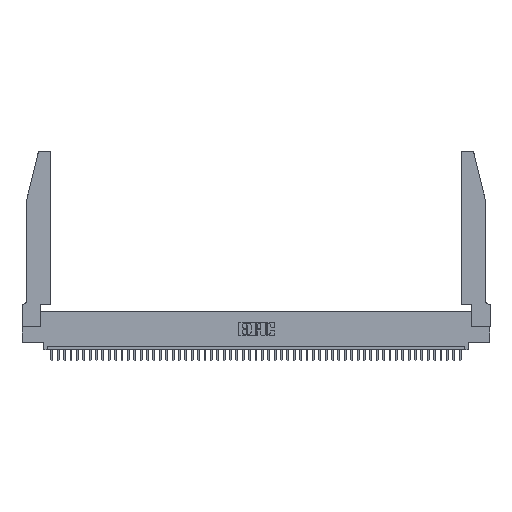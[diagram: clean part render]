
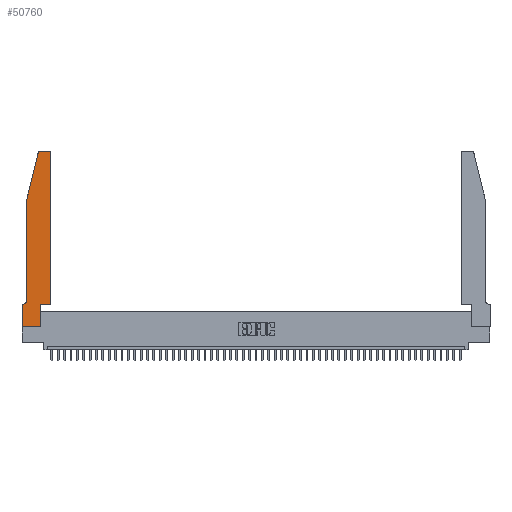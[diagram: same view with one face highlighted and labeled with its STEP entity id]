
A CAD part, top view. The second image highlights one B-rep face of the part: STEP entity #50760.
In plain terms, the highlighted planar face has unit normal (0, 0, 1).
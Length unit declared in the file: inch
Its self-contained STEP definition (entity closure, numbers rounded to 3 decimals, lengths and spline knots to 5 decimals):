
#1362 = CARTESIAN_POINT ( 'NONE',  ( 0.2605, 2.75, 0.37 ) ) ;
#1444 = AXIS2_PLACEMENT_3D ( 'NONE', #28934, #48845, #25145 ) ;
#1711 = CARTESIAN_POINT ( 'NONE',  ( 0.0055, 0.35, 0.37 ) ) ;
#2375 = VECTOR ( 'NONE', #44565, 39.37008 ) ;
#2603 = VERTEX_POINT ( 'NONE', #12487 ) ;
#3079 = VERTEX_POINT ( 'NONE', #20171 ) ;
#3161 = ORIENTED_EDGE ( 'NONE', *, *, #40107, .T. ) ;
#3470 = VECTOR ( 'NONE', #37490, 39.37008 ) ;
#3906 = VERTEX_POINT ( 'NONE', #20942 ) ;
#4210 = CARTESIAN_POINT ( 'NONE',  ( 0.25487, 2.72718, 0.37 ) ) ;
#4212 = ORIENTED_EDGE ( 'NONE', *, *, #50804, .T. ) ;
#4453 = ORIENTED_EDGE ( 'NONE', *, *, #38743, .T. ) ;
#4832 = DIRECTION ( 'NONE',  ( -0.239, -0.971, 0. ) ) ;
#5018 = CARTESIAN_POINT ( 'NONE',  ( 0.0755, 0.35, 0.37 ) ) ;
#5999 = LINE ( 'NONE', #22729, #45299 ) ;
#7219 = DIRECTION ( 'NONE',  ( 1., 0., 0. ) ) ;
#7527 = CARTESIAN_POINT ( 'NONE',  ( 0.2865, 0.35, 0.37 ) ) ;
#7775 = LINE ( 'NONE', #41407, #3470 ) ;
#7816 = VERTEX_POINT ( 'NONE', #7527 ) ;
#8596 = EDGE_CURVE ( 'NONE', #30933, #3079, #15545, .T. ) ;
#8912 = ORIENTED_EDGE ( 'NONE', *, *, #29137, .T. ) ;
#9221 = VERTEX_POINT ( 'NONE', #22425 ) ;
#9633 = CARTESIAN_POINT ( 'NONE',  ( 0.284, 2.72, 0.37 ) ) ;
#12421 = ORIENTED_EDGE ( 'NONE', *, *, #32654, .T. ) ;
#12487 = CARTESIAN_POINT ( 'NONE',  ( 0.2865, 0., 0.37 ) ) ;
#13029 = CARTESIAN_POINT ( 'NONE',  ( 0.4205, 2.72, 0.37 ) ) ;
#13188 = DIRECTION ( 'NONE',  ( 0., 0., 1. ) ) ;
#13356 = DIRECTION ( 'NONE',  ( 1., 0., 0. ) ) ;
#13885 = DIRECTION ( 'NONE',  ( 0., 0., 1. ) ) ;
#14765 = CARTESIAN_POINT ( 'NONE',  ( 0., 0.35, 0.37 ) ) ;
#14926 = EDGE_CURVE ( 'NONE', #9221, #30933, #44892, .T. ) ;
#15184 = DIRECTION ( 'NONE',  ( 0., -1., 0. ) ) ;
#15196 = VECTOR ( 'NONE', #15184, 39.37008 ) ;
#15411 = AXIS2_PLACEMENT_3D ( 'NONE', #9633, #13885, #41027 ) ;
#15545 = LINE ( 'NONE', #28526, #48084 ) ;
#15895 = VECTOR ( 'NONE', #19348, 39.37008 ) ;
#16087 = VERTEX_POINT ( 'NONE', #37648 ) ;
#16365 = DIRECTION ( 'NONE',  ( -1., 0., 0. ) ) ;
#16500 = LINE ( 'NONE', #1362, #29383 ) ;
#17758 = FACE_OUTER_BOUND ( 'NONE', #36509, .T. ) ;
#18768 = VERTEX_POINT ( 'NONE', #48513 ) ;
#18988 = DIRECTION ( 'NONE',  ( 0., 1., 0. ) ) ;
#19348 = DIRECTION ( 'NONE',  ( 1., 0., 0. ) ) ;
#19803 = ORIENTED_EDGE ( 'NONE', *, *, #22388, .T. ) ;
#20152 = VERTEX_POINT ( 'NONE', #38486 ) ;
#20171 = CARTESIAN_POINT ( 'NONE',  ( 0.0755, 2., 0.37 ) ) ;
#20942 = CARTESIAN_POINT ( 'NONE',  ( 0., 0.35, 0.37 ) ) ;
#21685 = LINE ( 'NONE', #42361, #37066 ) ;
#22388 = EDGE_CURVE ( 'NONE', #34232, #47552, #23246, .T. ) ;
#22425 = CARTESIAN_POINT ( 'NONE',  ( 0.284, 2.75, 0.37 ) ) ;
#22729 = CARTESIAN_POINT ( 'NONE',  ( 0.0755, 2., 0.37 ) ) ;
#23246 = LINE ( 'NONE', #36686, #2375 ) ;
#23311 = DIRECTION ( 'NONE',  ( 0., 0., 1. ) ) ;
#23414 = CARTESIAN_POINT ( 'NONE',  ( 0.4505, 2.72, 0.37 ) ) ;
#25145 = DIRECTION ( 'NONE',  ( -1., 0., 0. ) ) ;
#26842 = CARTESIAN_POINT ( 'NONE',  ( 0., 0., 0.37 ) ) ;
#27106 = PLANE ( 'NONE',  #31131 ) ;
#28047 = EDGE_CURVE ( 'NONE', #18768, #9221, #16500, .T. ) ;
#28526 = CARTESIAN_POINT ( 'NONE',  ( 0.0755, 2., 0.37 ) ) ;
#28934 = CARTESIAN_POINT ( 'NONE',  ( 0.0055, 0.42, 0.37 ) ) ;
#29137 = EDGE_CURVE ( 'NONE', #3906, #16087, #29869, .T. ) ;
#29383 = VECTOR ( 'NONE', #44754, 39.37008 ) ;
#29869 = LINE ( 'NONE', #26842, #15196 ) ;
#30098 = ORIENTED_EDGE ( 'NONE', *, *, #8596, .T. ) ;
#30838 = ORIENTED_EDGE ( 'NONE', *, *, #46877, .T. ) ;
#30933 = VERTEX_POINT ( 'NONE', #4210 ) ;
#31131 = AXIS2_PLACEMENT_3D ( 'NONE', #14765, #23311, #7219 ) ;
#31739 = CIRCLE ( 'NONE', #44949, 0.03 ) ;
#31907 = LINE ( 'NONE', #5018, #42383 ) ;
#32654 = EDGE_CURVE ( 'NONE', #47552, #18768, #31739, .T. ) ;
#34232 = VERTEX_POINT ( 'NONE', #38812 ) ;
#34559 = DIRECTION ( 'NONE',  ( 0., -1., 0. ) ) ;
#35914 = ORIENTED_EDGE ( 'NONE', *, *, #28047, .T. ) ;
#36509 = EDGE_LOOP ( 'NONE', ( #35914, #39412, #30098, #30838, #3161, #4453, #8912, #43967, #37861, #4212, #19803, #12421 ) ) ;
#36686 = CARTESIAN_POINT ( 'NONE',  ( 0.4505, 0.35, 0.37 ) ) ;
#37066 = VECTOR ( 'NONE', #18988, 39.37008 ) ;
#37326 = EDGE_CURVE ( 'NONE', #2603, #7816, #21685, .T. ) ;
#37490 = DIRECTION ( 'NONE',  ( 1., 0., 0. ) ) ;
#37648 = CARTESIAN_POINT ( 'NONE',  ( 0., 0., 0.37 ) ) ;
#37861 = ORIENTED_EDGE ( 'NONE', *, *, #37326, .T. ) ;
#38486 = CARTESIAN_POINT ( 'NONE',  ( 0.0755, 0.42, 0.37 ) ) ;
#38743 = EDGE_CURVE ( 'NONE', #48579, #3906, #31907, .T. ) ;
#38812 = CARTESIAN_POINT ( 'NONE',  ( 0.4505, 0.35, 0.37 ) ) ;
#38981 = CARTESIAN_POINT ( 'NONE',  ( 0.4505, 0.35, 0.37 ) ) ;
#39412 = ORIENTED_EDGE ( 'NONE', *, *, #14926, .T. ) ;
#40107 = EDGE_CURVE ( 'NONE', #20152, #48579, #45900, .T. ) ;
#40837 = EDGE_CURVE ( 'NONE', #16087, #2603, #7775, .T. ) ;
#41027 = DIRECTION ( 'NONE',  ( 1., 0., 0. ) ) ;
#41407 = CARTESIAN_POINT ( 'NONE',  ( 0., 0., 0.37 ) ) ;
#42361 = CARTESIAN_POINT ( 'NONE',  ( 0.2865, 0.35, 0.37 ) ) ;
#42383 = VECTOR ( 'NONE', #16365, 39.37008 ) ;
#43967 = ORIENTED_EDGE ( 'NONE', *, *, #40837, .T. ) ;
#44565 = DIRECTION ( 'NONE',  ( 0., 1., 0. ) ) ;
#44754 = DIRECTION ( 'NONE',  ( -1., 0., 0. ) ) ;
#44892 = CIRCLE ( 'NONE', #15411, 0.03 ) ;
#44949 = AXIS2_PLACEMENT_3D ( 'NONE', #13029, #13188, #13356 ) ;
#45299 = VECTOR ( 'NONE', #34559, 39.37008 ) ;
#45900 = CIRCLE ( 'NONE', #1444, 0.07 ) ;
#46877 = EDGE_CURVE ( 'NONE', #3079, #20152, #5999, .T. ) ;
#47552 = VERTEX_POINT ( 'NONE', #23414 ) ;
#48084 = VECTOR ( 'NONE', #4832, 39.37008 ) ;
#48513 = CARTESIAN_POINT ( 'NONE',  ( 0.4205, 2.75, 0.37 ) ) ;
#48579 = VERTEX_POINT ( 'NONE', #1711 ) ;
#48845 = DIRECTION ( 'NONE',  ( 0., 0., -1. ) ) ;
#49656 = LINE ( 'NONE', #38981, #15895 ) ;
#50760 = ADVANCED_FACE ( 'NONE', ( #17758 ), #27106, .T. ) ;
#50804 = EDGE_CURVE ( 'NONE', #7816, #34232, #49656, .T. ) ;
